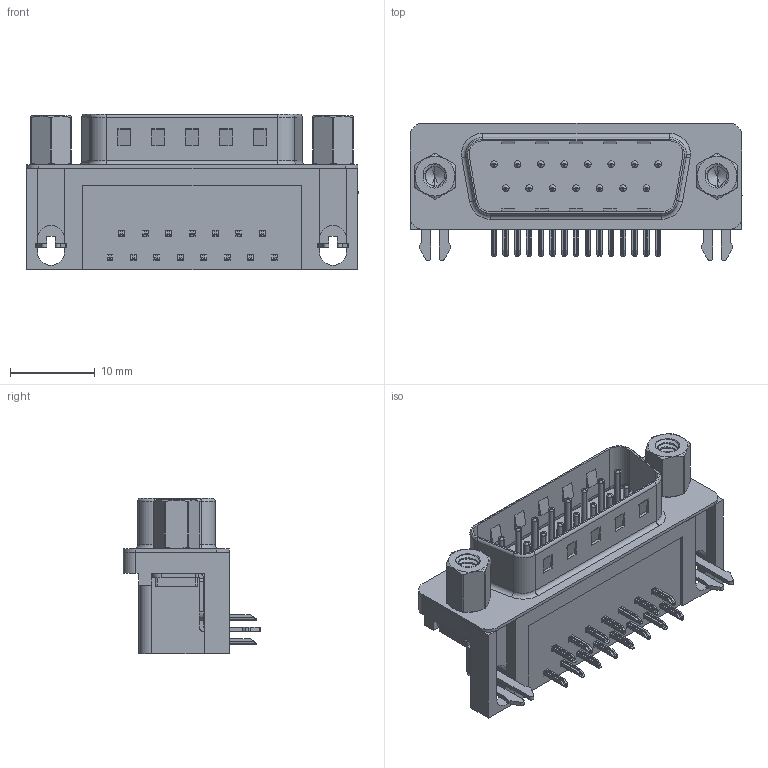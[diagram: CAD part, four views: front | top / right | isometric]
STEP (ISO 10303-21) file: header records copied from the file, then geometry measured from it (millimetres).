
FILE_DESCRIPTION (( 'STEP AP203' ), '1' );
FILE_NAME ('621-015-368-533.STEP', '2019-11-19T00:56:18', ( '' ), ( '' ), 'SwSTEP 2.0', 'SolidWorks 2016', '' );
FILE_SCHEMA (( 'CONFIG_CONTROL_DESIGN' ));
Length unit declared in the file: millimetre
Products named in the file (8): 621 2 Prong Board Lock; 621-015-368-533; 621 Housing_15 Socket; 621 Contact Bottom; 621 4-40 Threaded Rivet; 621 Shell_15 Socket; 621 Contact Top; 621 4-40 Hex Standoff 5
Assembly tree (23 placements, depth 2):
  621-015-368-533
    621 Housing_15 Socket
    621 Shell_15 Socket
    621 Contact Bottom  x7
    621 Contact Top  x8
    621 2 Prong Board Lock  x2
    621 4-40 Threaded Rivet  x2
    621 4-40 Hex Standoff 5  x2
Bounding box: 39.22 x 16.25 x 18.4 mm (x, y, z)
Volume: 4627.6 mm3; surface area: 6138.8 mm2
Topology: 23 solids, 23 shells, 1643 faces, 4147 edges, 2587 vertices
Faces by surface type: plane 947, cylinder 525, torus 121, cone 32, bspline 18
Entity records: 24360 total; most frequent: CARTESIAN_POINT 7936, ORIENTED_EDGE 3168, DIRECTION 3149, EDGE_CURVE 1584, AXIS2_PLACEMENT_3D 1064, VECTOR 1021, LINE 1021, VERTEX_POINT 1016
